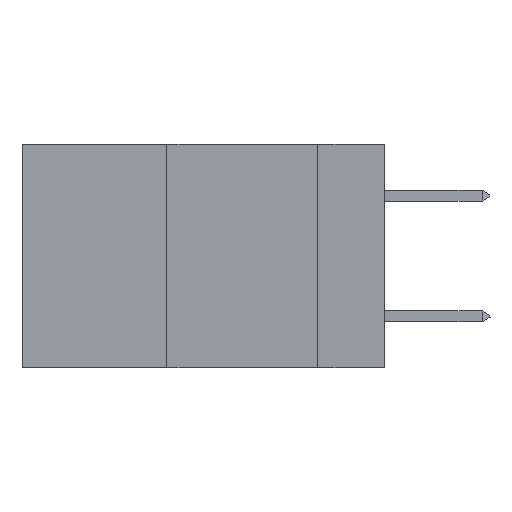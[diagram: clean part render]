
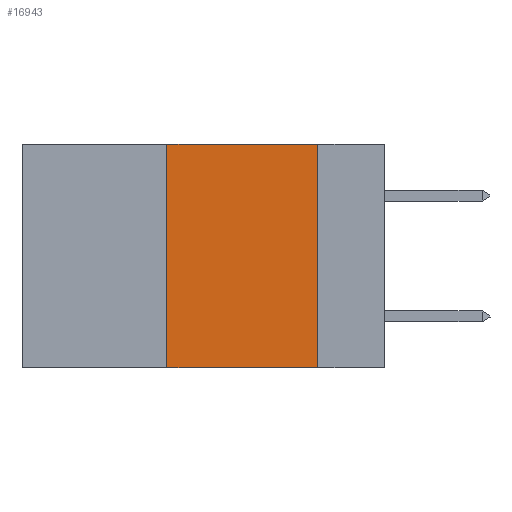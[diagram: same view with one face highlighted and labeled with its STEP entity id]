
A CAD part, left-side view. The second image highlights one B-rep face of the part: STEP entity #16943.
In plain terms, the highlighted planar face has unit normal (-1, 0, 0).
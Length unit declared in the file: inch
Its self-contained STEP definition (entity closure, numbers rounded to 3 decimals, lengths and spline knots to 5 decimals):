
#2027 = ORIENTED_EDGE ( 'NONE', *, *, #15433, .T. ) ;
#2266 = DIRECTION ( 'NONE',  ( 1., 0., 0. ) ) ;
#2552 = FACE_OUTER_BOUND ( 'NONE', #10580, .T. ) ;
#5493 = ORIENTED_EDGE ( 'NONE', *, *, #26891, .F. ) ;
#6527 = ORIENTED_EDGE ( 'NONE', *, *, #21910, .F. ) ;
#6890 = CARTESIAN_POINT ( 'NONE',  ( 0., 0.11, 0. ) ) ;
#8369 = EDGE_CURVE ( 'NONE', #8624, #23226, #25663, .T. ) ;
#8624 = VERTEX_POINT ( 'NONE', #26603 ) ;
#9932 = VECTOR ( 'NONE', #12300, 39.37008 ) ;
#10580 = EDGE_LOOP ( 'NONE', ( #27076, #6527, #5493, #2027 ) ) ;
#10649 = CARTESIAN_POINT ( 'NONE',  ( 0., 0.6, 0. ) ) ;
#10689 = VECTOR ( 'NONE', #23662, 39.37008 ) ;
#11020 = DIRECTION ( 'NONE',  ( 0., 0., -1. ) ) ;
#11589 = DIRECTION ( 'NONE',  ( 0., -1., 0. ) ) ;
#12234 = CARTESIAN_POINT ( 'NONE',  ( 0., 0.11, -0.37 ) ) ;
#12300 = DIRECTION ( 'NONE',  ( 0., -1., 0. ) ) ;
#12470 = VECTOR ( 'NONE', #11589, 39.37008 ) ;
#12788 = PLANE ( 'NONE',  #17093 ) ;
#13596 = DIRECTION ( 'NONE',  ( 0., 0., -1. ) ) ;
#13621 = VERTEX_POINT ( 'NONE', #25094 ) ;
#14330 = LINE ( 'NONE', #23479, #10689 ) ;
#15433 = EDGE_CURVE ( 'NONE', #16578, #23226, #16407, .T. ) ;
#16407 = LINE ( 'NONE', #21831, #12470 ) ;
#16578 = VERTEX_POINT ( 'NONE', #22307 ) ;
#16943 = ADVANCED_FACE ( 'NONE', ( #2552 ), #12788, .F. ) ;
#17058 = VECTOR ( 'NONE', #13596, 39.37008 ) ;
#17093 = AXIS2_PLACEMENT_3D ( 'NONE', #10649, #2266, #11020 ) ;
#20189 = LINE ( 'NONE', #27244, #9932 ) ;
#21831 = CARTESIAN_POINT ( 'NONE',  ( 0., 0.6, -0.37 ) ) ;
#21910 = EDGE_CURVE ( 'NONE', #13621, #8624, #20189, .T. ) ;
#22307 = CARTESIAN_POINT ( 'NONE',  ( 0., 0.36, -0.37 ) ) ;
#23226 = VERTEX_POINT ( 'NONE', #12234 ) ;
#23479 = CARTESIAN_POINT ( 'NONE',  ( 0., 0.36, 0. ) ) ;
#23662 = DIRECTION ( 'NONE',  ( 0., 0., 1. ) ) ;
#25094 = CARTESIAN_POINT ( 'NONE',  ( 0., 0.36, 0. ) ) ;
#25663 = LINE ( 'NONE', #6890, #17058 ) ;
#26603 = CARTESIAN_POINT ( 'NONE',  ( 0., 0.11, 0. ) ) ;
#26891 = EDGE_CURVE ( 'NONE', #16578, #13621, #14330, .T. ) ;
#27076 = ORIENTED_EDGE ( 'NONE', *, *, #8369, .F. ) ;
#27244 = CARTESIAN_POINT ( 'NONE',  ( 0., 0.6, 0. ) ) ;
